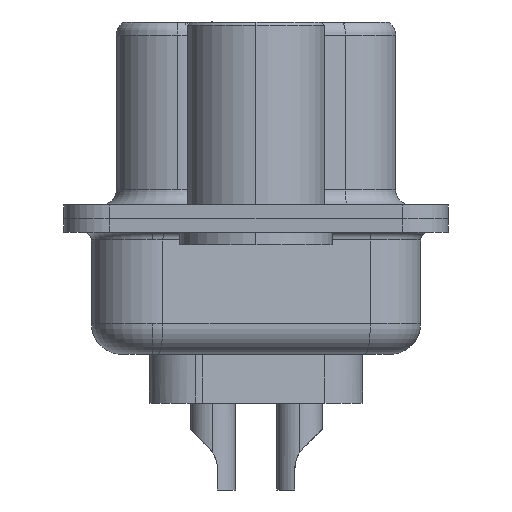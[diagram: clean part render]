
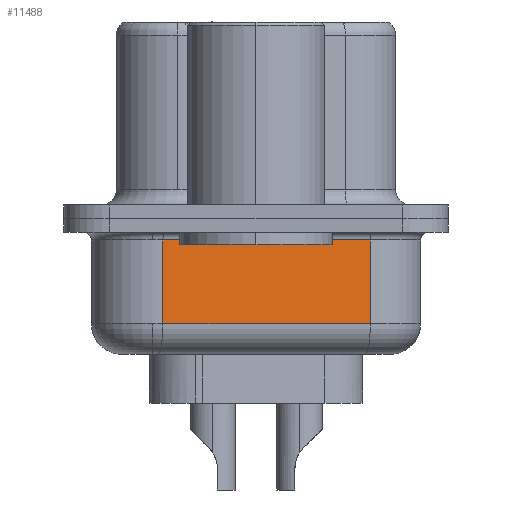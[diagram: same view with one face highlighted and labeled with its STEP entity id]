
A CAD part, left-side view. The second image highlights one B-rep face of the part: STEP entity #11488.
In plain terms, the highlighted planar face has unit normal (-0.985, -0.174, 0).
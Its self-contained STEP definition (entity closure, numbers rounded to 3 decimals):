
#262 = EDGE_CURVE ( 'NONE', #3042, #7110, #2899, .T. ) ;
#1270 = EDGE_CURVE ( 'NONE', #11464, #7110, #26352, .T. ) ;
#1423 = LINE ( 'NONE', #15750, #12204 ) ;
#2224 = VECTOR ( 'NONE', #24860, 1000. ) ;
#2682 = DIRECTION ( 'NONE',  ( 0.174, -0.985, 0. ) ) ;
#2827 = DIRECTION ( 'NONE',  ( 0., 0., 1. ) ) ;
#2899 = LINE ( 'NONE', #11061, #2224 ) ;
#3042 = VERTEX_POINT ( 'NONE', #24272 ) ;
#4055 = CARTESIAN_POINT ( 'NONE',  ( 4.079, -3.747, -3.45 ) ) ;
#4805 = CARTESIAN_POINT ( 'NONE',  ( 2.88, 3.053, -4.45 ) ) ;
#6975 = PLANE ( 'NONE',  #22048 ) ;
#7085 = ORIENTED_EDGE ( 'NONE', *, *, #262, .T. ) ;
#7110 = VERTEX_POINT ( 'NONE', #26863 ) ;
#7237 = ORIENTED_EDGE ( 'NONE', *, *, #8744, .T. ) ;
#8744 = EDGE_CURVE ( 'NONE', #11464, #17795, #27691, .T. ) ;
#9115 = DIRECTION ( 'NONE',  ( 0.985, 0.174, 0. ) ) ;
#9427 = EDGE_CURVE ( 'NONE', #17795, #3042, #1423, .T. ) ;
#10581 = VECTOR ( 'NONE', #2682, 1000. ) ;
#11061 = CARTESIAN_POINT ( 'NONE',  ( 2.88, 3.053, -0.7 ) ) ;
#11464 = VERTEX_POINT ( 'NONE', #17522 ) ;
#11488 = ADVANCED_FACE ( 'NONE', ( #12191 ), #6975, .F. ) ;
#12191 = FACE_OUTER_BOUND ( 'NONE', #22309, .T. ) ;
#12204 = VECTOR ( 'NONE', #2827, 1000. ) ;
#14906 = VECTOR ( 'NONE', #23160, 1000. ) ;
#15663 = ORIENTED_EDGE ( 'NONE', *, *, #9427, .T. ) ;
#15750 = CARTESIAN_POINT ( 'NONE',  ( 4.079, -3.747, -4.45 ) ) ;
#17116 = CARTESIAN_POINT ( 'NONE',  ( 2.88, 3.053, -4.45 ) ) ;
#17522 = CARTESIAN_POINT ( 'NONE',  ( 2.88, 3.053, -3.45 ) ) ;
#17701 = ORIENTED_EDGE ( 'NONE', *, *, #1270, .F. ) ;
#17795 = VERTEX_POINT ( 'NONE', #4055 ) ;
#22048 = AXIS2_PLACEMENT_3D ( 'NONE', #4805, #9115, #24114 ) ;
#22309 = EDGE_LOOP ( 'NONE', ( #17701, #7237, #15663, #7085 ) ) ;
#23160 = DIRECTION ( 'NONE',  ( 0., 0., 1. ) ) ;
#24114 = DIRECTION ( 'NONE',  ( -0.174, 0.985, 0. ) ) ;
#24272 = CARTESIAN_POINT ( 'NONE',  ( 4.079, -3.747, -0.7 ) ) ;
#24860 = DIRECTION ( 'NONE',  ( -0.174, 0.985, 0. ) ) ;
#26248 = CARTESIAN_POINT ( 'NONE',  ( 2.88, 3.053, -3.45 ) ) ;
#26352 = LINE ( 'NONE', #17116, #14906 ) ;
#26863 = CARTESIAN_POINT ( 'NONE',  ( 2.88, 3.053, -0.7 ) ) ;
#27691 = LINE ( 'NONE', #26248, #10581 ) ;
